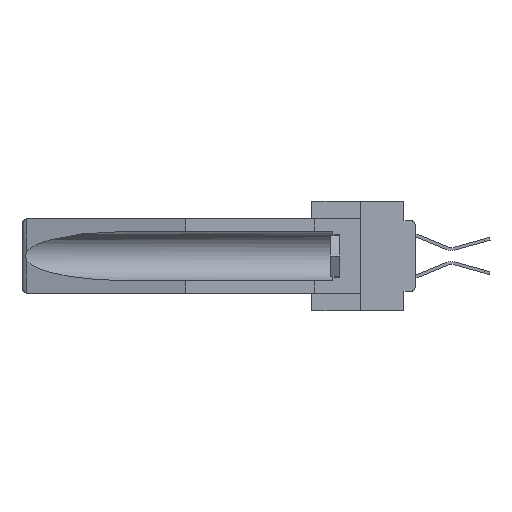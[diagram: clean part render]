
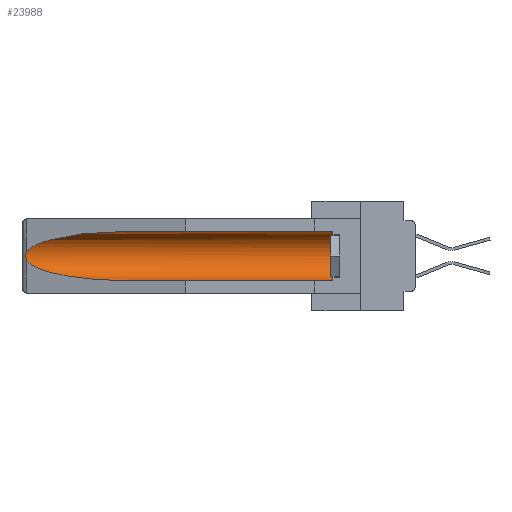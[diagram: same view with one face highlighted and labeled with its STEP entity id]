
A CAD part, left-side view. The second image highlights one B-rep face of the part: STEP entity #23988.
In plain terms, the highlighted cylindrical face has radius 2.857 mm (diameter 5.715 mm), a partial arc.
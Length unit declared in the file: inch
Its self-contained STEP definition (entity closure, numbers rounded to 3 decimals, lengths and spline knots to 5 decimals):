
#354 = DIRECTION ( 'NONE',  ( 0., -1., 0. ) ) ;
#898 = ORIENTED_EDGE ( 'NONE', *, *, #20578, .T. ) ;
#1376 = VERTEX_POINT ( 'NONE', #25554 ) ;
#1605 = CARTESIAN_POINT ( 'NONE',  ( 0.2675, 1.53308, -0.16763 ) ) ;
#1812 = CARTESIAN_POINT ( 'NONE',  ( 0.26597, 1.52961, -0.15275 ) ) ;
#2938 = FACE_OUTER_BOUND ( 'NONE', #27427, .T. ) ;
#3059 = DIRECTION ( 'NONE',  ( 0., 1., 0. ) ) ;
#3237 = ORIENTED_EDGE ( 'NONE', *, *, #6600, .F. ) ;
#3278 = VERTEX_POINT ( 'NONE', #25454 ) ;
#3281 = CARTESIAN_POINT ( 'NONE',  ( 0.155, -0.30754, -0.059 ) ) ;
#3869 = CARTESIAN_POINT ( 'NONE',  ( 0.155, 1.07973, -0.059 ) ) ;
#4257 = VERTEX_POINT ( 'NONE', #18768 ) ;
#5661 = AXIS2_PLACEMENT_3D ( 'NONE', #25571, #16256, #20989 ) ;
#6462 = CARTESIAN_POINT ( 'NONE',  ( 0.26597, 1.5296, -0.19026 ) ) ;
#6600 = EDGE_CURVE ( 'NONE', #4257, #21839, #20157, .T. ) ;
#6655 = CARTESIAN_POINT ( 'NONE',  ( 0.155, 1.07973, -0.284 ) ) ;
#6913 = CYLINDRICAL_SURFACE ( 'NONE', #5661, 0.1125 ) ;
#6977 = EDGE_CURVE ( 'NONE', #21709, #21839, #29185, .T. ) ;
#7461 = CARTESIAN_POINT ( 'NONE',  ( 0.155, 0.126, -0.1715 ) ) ;
#8478 = CARTESIAN_POINT ( 'NONE',  ( 0.25451, 1.48313, -0.09465 ) ) ;
#8768 = CARTESIAN_POINT ( 'NONE',  ( 0.26537, 1.52718, -0.19328 ) ) ;
#8939 = EDGE_CURVE ( 'NONE', #16404, #3278, #23725, .T. ) ;
#10701 = CARTESIAN_POINT ( 'NONE',  ( 0.26537, 1.52718, -0.14972 ) ) ;
#11058 = ORIENTED_EDGE ( 'NONE', *, *, #12958, .T. ) ;
#11436 = CIRCLE ( 'NONE', #14844, 0.1125 ) ;
#12958 = EDGE_CURVE ( 'NONE', #3278, #1376, #22528, .T. ) ;
#13417 = ORIENTED_EDGE ( 'NONE', *, *, #8939, .T. ) ;
#14005 = VECTOR ( 'NONE', #19233, 39.37008 ) ;
#14574 = CARTESIAN_POINT ( 'NONE',  ( 0.155, -0.30754, -0.284 ) ) ;
#14651 = VECTOR ( 'NONE', #3059, 39.37008 ) ;
#14844 = AXIS2_PLACEMENT_3D ( 'NONE', #7461, #354, #23558 ) ;
#16256 = DIRECTION ( 'NONE',  ( 0., 1., 0. ) ) ;
#16404 = VERTEX_POINT ( 'NONE', #28668 ) ;
#16601 = ORIENTED_EDGE ( 'NONE', *, *, #19044, .T. ) ;
#18091 = CARTESIAN_POINT ( 'NONE',  ( 0.21114, 1.30732, -0.284 ) ) ;
#18768 = CARTESIAN_POINT ( 'NONE',  ( 0.155, 0.126, -0.284 ) ) ;
#18781 = CARTESIAN_POINT ( 'NONE',  ( 0.26537, 1.52718, -0.19328 ) ) ;
#19044 = EDGE_CURVE ( 'NONE', #4257, #16404, #11436, .T. ) ;
#19233 = DIRECTION ( 'NONE',  ( 0., 1., 0. ) ) ;
#20007 = CARTESIAN_POINT ( 'NONE',  ( 0.21114, 1.30732, -0.059 ) ) ;
#20157 = LINE ( 'NONE', #14574, #14005 ) ;
#20192 = CARTESIAN_POINT ( 'NONE',  ( 0.26654, 1.53092, -0.15636 ) ) ;
#20578 = EDGE_CURVE ( 'NONE', #1376, #21709, #20655, .T. ) ;
#20655 = B_SPLINE_CURVE_WITH_KNOTS ( 'NONE', 3,
 ( #10701, #1812, #20192, #29188, #1605, #22449, #27193, #24658, #6462, #22631 ),
 .UNSPECIFIED., .F., .F.,
 ( 4, 2, 2, 2, 4 ),
 ( 0., 0.00029, 0.00058, 0.00087, 0.00117 ),
 .UNSPECIFIED. ) ;
#20989 = DIRECTION ( 'NONE',  ( 0., 0., 1. ) ) ;
#21709 = VERTEX_POINT ( 'NONE', #18781 ) ;
#21839 = VERTEX_POINT ( 'NONE', #23473 ) ;
#22449 = CARTESIAN_POINT ( 'NONE',  ( 0.2675, 1.53308, -0.17534 ) ) ;
#22528 =( BOUNDED_CURVE ( )  B_SPLINE_CURVE ( 3, ( #3869, #20007, #8478, #29318 ),
 .UNSPECIFIED., .F., .F. ) 
 B_SPLINE_CURVE_WITH_KNOTS ( ( 4, 4 ),
 ( 4.71239, 6.08839 ),
 .UNSPECIFIED. ) 
 CURVE ( )  GEOMETRIC_REPRESENTATION_ITEM ( )  RATIONAL_B_SPLINE_CURVE ( ( 1., 0.848, 0.848, 1. ) ) 
 REPRESENTATION_ITEM ( '' )  );
#22631 = CARTESIAN_POINT ( 'NONE',  ( 0.26537, 1.52718, -0.19328 ) ) ;
#23473 = CARTESIAN_POINT ( 'NONE',  ( 0.155, 1.07973, -0.284 ) ) ;
#23558 = DIRECTION ( 'NONE',  ( 0., 0., 1. ) ) ;
#23725 = LINE ( 'NONE', #3281, #14651 ) ;
#23988 = ADVANCED_FACE ( 'NONE', ( #2938 ), #6913, .F. ) ;
#24658 = CARTESIAN_POINT ( 'NONE',  ( 0.26655, 1.53094, -0.18657 ) ) ;
#25454 = CARTESIAN_POINT ( 'NONE',  ( 0.155, 1.07973, -0.059 ) ) ;
#25554 = CARTESIAN_POINT ( 'NONE',  ( 0.26537, 1.52718, -0.14972 ) ) ;
#25571 = CARTESIAN_POINT ( 'NONE',  ( 0.155, -0.30754, -0.1715 ) ) ;
#27193 = CARTESIAN_POINT ( 'NONE',  ( 0.2673, 1.53269, -0.17917 ) ) ;
#27427 = EDGE_LOOP ( 'NONE', ( #11058, #898, #29290, #3237, #16601, #13417 ) ) ;
#27584 = CARTESIAN_POINT ( 'NONE',  ( 0.25451, 1.48313, -0.24835 ) ) ;
#28668 = CARTESIAN_POINT ( 'NONE',  ( 0.155, 0.126, -0.059 ) ) ;
#29185 =( BOUNDED_CURVE ( )  B_SPLINE_CURVE ( 3, ( #8768, #27584, #18091, #6655 ),
 .UNSPECIFIED., .F., .F. ) 
 B_SPLINE_CURVE_WITH_KNOTS ( ( 4, 4 ),
 ( 0.1948, 1.5708 ),
 .UNSPECIFIED. ) 
 CURVE ( )  GEOMETRIC_REPRESENTATION_ITEM ( )  RATIONAL_B_SPLINE_CURVE ( ( 1., 0.848, 0.848, 1. ) ) 
 REPRESENTATION_ITEM ( '' )  );
#29188 = CARTESIAN_POINT ( 'NONE',  ( 0.2673, 1.5327, -0.16383 ) ) ;
#29290 = ORIENTED_EDGE ( 'NONE', *, *, #6977, .T. ) ;
#29318 = CARTESIAN_POINT ( 'NONE',  ( 0.26537, 1.52718, -0.14972 ) ) ;
